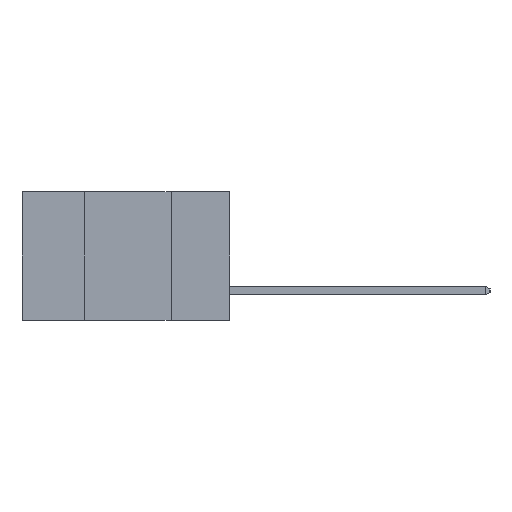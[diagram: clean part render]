
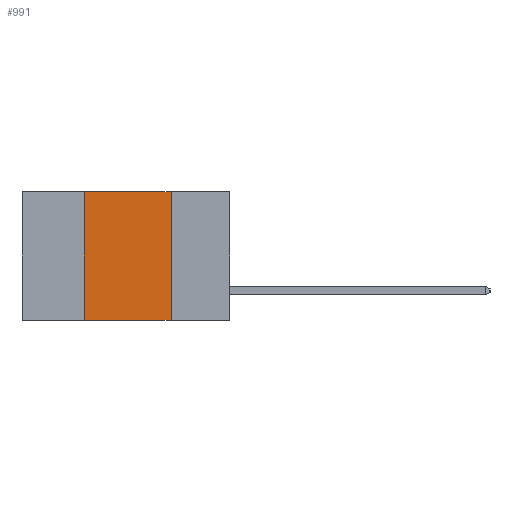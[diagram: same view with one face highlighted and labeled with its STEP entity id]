
A CAD part, left-side view. The second image highlights one B-rep face of the part: STEP entity #991.
In plain terms, the highlighted planar face has unit normal (-1, 0, 0).
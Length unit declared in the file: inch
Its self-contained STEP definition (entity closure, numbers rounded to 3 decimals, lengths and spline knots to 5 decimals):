
#915 = DIRECTION ( 'NONE',  ( 1., 0., 0. ) ) ;
#991 = ADVANCED_FACE ( 'NONE', ( #9102 ), #1068, .F. ) ;
#1068 = PLANE ( 'NONE',  #8884 ) ;
#1169 = ORIENTED_EDGE ( 'NONE', *, *, #5836, .F. ) ;
#1267 = VECTOR ( 'NONE', #1397, 39.37008 ) ;
#1293 = VERTEX_POINT ( 'NONE', #8694 ) ;
#1331 = CARTESIAN_POINT ( 'NONE',  ( 0., 0.6, -0.37 ) ) ;
#1345 = CARTESIAN_POINT ( 'NONE',  ( 0., 0.42, 0. ) ) ;
#1397 = DIRECTION ( 'NONE',  ( 0., 0., -1. ) ) ;
#1531 = VERTEX_POINT ( 'NONE', #3988 ) ;
#1961 = CARTESIAN_POINT ( 'NONE',  ( 0., 0.42, 0. ) ) ;
#2382 = ORIENTED_EDGE ( 'NONE', *, *, #8508, .F. ) ;
#3436 = ORIENTED_EDGE ( 'NONE', *, *, #5793, .T. ) ;
#3933 = CARTESIAN_POINT ( 'NONE',  ( 0., 0.6, 0. ) ) ;
#3988 = CARTESIAN_POINT ( 'NONE',  ( 0., 0.17, -0.37 ) ) ;
#4096 = CARTESIAN_POINT ( 'NONE',  ( 0., 0.6, 0. ) ) ;
#4113 = ORIENTED_EDGE ( 'NONE', *, *, #6818, .F. ) ;
#4336 = VERTEX_POINT ( 'NONE', #6594 ) ;
#4358 = DIRECTION ( 'NONE',  ( 0., -1., 0. ) ) ;
#4386 = VERTEX_POINT ( 'NONE', #1345 ) ;
#4593 = VECTOR ( 'NONE', #5593, 39.37008 ) ;
#5593 = DIRECTION ( 'NONE',  ( 0., 0., 1. ) ) ;
#5793 = EDGE_CURVE ( 'NONE', #1293, #1531, #7413, .T. ) ;
#5836 = EDGE_CURVE ( 'NONE', #4336, #1531, #8904, .T. ) ;
#6594 = CARTESIAN_POINT ( 'NONE',  ( 0., 0.17, 0. ) ) ;
#6818 = EDGE_CURVE ( 'NONE', #4386, #4336, #8892, .T. ) ;
#6914 = DIRECTION ( 'NONE',  ( 0., 0., -1. ) ) ;
#7162 = LINE ( 'NONE', #1961, #4593 ) ;
#7413 = LINE ( 'NONE', #1331, #9082 ) ;
#7789 = DIRECTION ( 'NONE',  ( 0., -1., 0. ) ) ;
#8145 = EDGE_LOOP ( 'NONE', ( #1169, #4113, #2382, #3436 ) ) ;
#8232 = CARTESIAN_POINT ( 'NONE',  ( 0., 0.17, 0. ) ) ;
#8508 = EDGE_CURVE ( 'NONE', #1293, #4386, #7162, .T. ) ;
#8694 = CARTESIAN_POINT ( 'NONE',  ( 0., 0.42, -0.37 ) ) ;
#8699 = VECTOR ( 'NONE', #7789, 39.37008 ) ;
#8884 = AXIS2_PLACEMENT_3D ( 'NONE', #3933, #915, #6914 ) ;
#8892 = LINE ( 'NONE', #4096, #8699 ) ;
#8904 = LINE ( 'NONE', #8232, #1267 ) ;
#9082 = VECTOR ( 'NONE', #4358, 39.37008 ) ;
#9102 = FACE_OUTER_BOUND ( 'NONE', #8145, .T. ) ;
